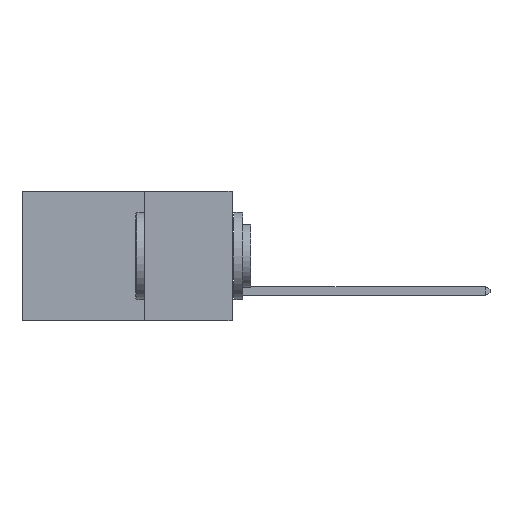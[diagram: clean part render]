
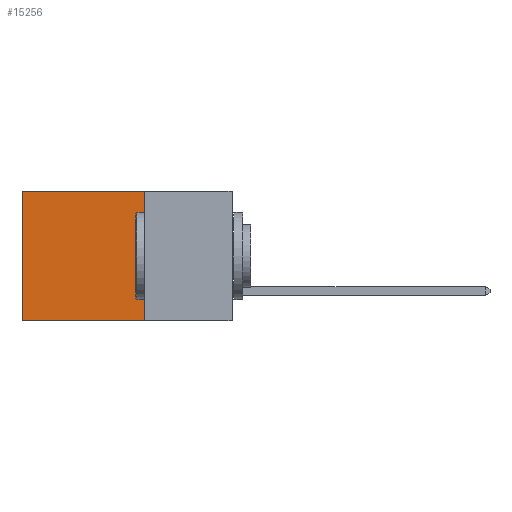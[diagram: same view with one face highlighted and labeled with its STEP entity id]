
A CAD part, left-side view. The second image highlights one B-rep face of the part: STEP entity #15256.
In plain terms, the highlighted planar face has unit normal (-1, 0, 0).
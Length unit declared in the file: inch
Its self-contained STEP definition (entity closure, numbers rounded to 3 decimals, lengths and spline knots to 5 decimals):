
#5 = CARTESIAN_POINT ( 'NONE',  ( 0.2875, 0.6, 0. ) ) ;
#192 = ORIENTED_EDGE ( 'NONE', *, *, #15942, .T. ) ;
#259 = CARTESIAN_POINT ( 'NONE',  ( 0.2875, 0.25, -0.37 ) ) ;
#779 = PLANE ( 'NONE',  #18934 ) ;
#1226 = DIRECTION ( 'NONE',  ( 0., 1., 0. ) ) ;
#1279 = CARTESIAN_POINT ( 'NONE',  ( 0.2875, 0.6, -0.37 ) ) ;
#1774 = CARTESIAN_POINT ( 'NONE',  ( 0.2875, 0.6, 0. ) ) ;
#2365 = DIRECTION ( 'NONE',  ( 0., 0., -1. ) ) ;
#2441 = VECTOR ( 'NONE', #8258, 39.37008 ) ;
#2558 = VERTEX_POINT ( 'NONE', #1279 ) ;
#2792 = CARTESIAN_POINT ( 'NONE',  ( 0.2875, 0.25, 0. ) ) ;
#2821 = EDGE_CURVE ( 'NONE', #17326, #2558, #16249, .T. ) ;
#3382 = LINE ( 'NONE', #8452, #2441 ) ;
#3730 = VECTOR ( 'NONE', #17794, 39.37008 ) ;
#4192 = VECTOR ( 'NONE', #1226, 39.37008 ) ;
#4670 = LINE ( 'NONE', #2792, #4192 ) ;
#5192 = VERTEX_POINT ( 'NONE', #18814 ) ;
#7050 = EDGE_LOOP ( 'NONE', ( #17576, #15353, #15465, #192 ) ) ;
#8258 = DIRECTION ( 'NONE',  ( 0., 0., -1. ) ) ;
#8452 = CARTESIAN_POINT ( 'NONE',  ( 0.2875, 0.25, 0. ) ) ;
#8996 = FACE_OUTER_BOUND ( 'NONE', #7050, .T. ) ;
#11509 = DIRECTION ( 'NONE',  ( 1., 0., 0. ) ) ;
#12053 = EDGE_CURVE ( 'NONE', #5192, #17326, #3382, .T. ) ;
#12553 = VERTEX_POINT ( 'NONE', #1774 ) ;
#13785 = DIRECTION ( 'NONE',  ( 0., 1., 0. ) ) ;
#13861 = CARTESIAN_POINT ( 'NONE',  ( 0.2875, 0.25, -0.37 ) ) ;
#15256 = ADVANCED_FACE ( 'NONE', ( #8996 ), #779, .F. ) ;
#15353 = ORIENTED_EDGE ( 'NONE', *, *, #2821, .F. ) ;
#15465 = ORIENTED_EDGE ( 'NONE', *, *, #12053, .F. ) ;
#15526 = EDGE_CURVE ( 'NONE', #12553, #2558, #15626, .T. ) ;
#15626 = LINE ( 'NONE', #5, #3730 ) ;
#15794 = VECTOR ( 'NONE', #13785, 39.37008 ) ;
#15942 = EDGE_CURVE ( 'NONE', #5192, #12553, #4670, .T. ) ;
#16249 = LINE ( 'NONE', #13861, #15794 ) ;
#17145 = CARTESIAN_POINT ( 'NONE',  ( 0.2875, 0.25, 0. ) ) ;
#17326 = VERTEX_POINT ( 'NONE', #259 ) ;
#17576 = ORIENTED_EDGE ( 'NONE', *, *, #15526, .T. ) ;
#17794 = DIRECTION ( 'NONE',  ( 0., 0., -1. ) ) ;
#18814 = CARTESIAN_POINT ( 'NONE',  ( 0.2875, 0.25, 0. ) ) ;
#18934 = AXIS2_PLACEMENT_3D ( 'NONE', #17145, #11509, #2365 ) ;
